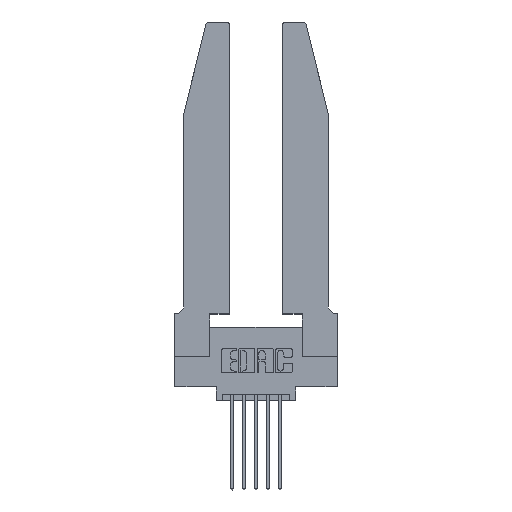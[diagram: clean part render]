
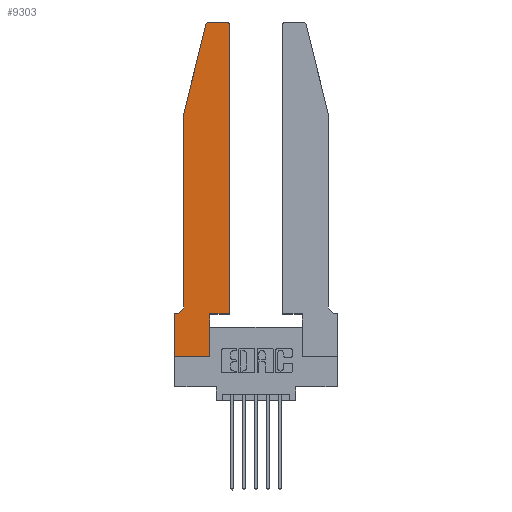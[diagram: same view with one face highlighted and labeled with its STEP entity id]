
A CAD part, top view. The second image highlights one B-rep face of the part: STEP entity #9303.
In plain terms, the highlighted planar face has unit normal (0, 0, 1).
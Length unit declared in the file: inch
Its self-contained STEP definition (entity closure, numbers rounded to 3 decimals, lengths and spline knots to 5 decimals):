
#86 = VECTOR ( 'NONE', #9740, 39.37008 ) ;
#114 = DIRECTION ( 'NONE',  ( 1., 0., 0. ) ) ;
#290 = AXIS2_PLACEMENT_3D ( 'NONE', #9185, #13426, #3967 ) ;
#351 = ORIENTED_EDGE ( 'NONE', *, *, #12800, .T. ) ;
#453 = DIRECTION ( 'NONE',  ( -0.239, -0.971, 0. ) ) ;
#692 = DIRECTION ( 'NONE',  ( -1., 0., 0. ) ) ;
#730 = DIRECTION ( 'NONE',  ( 0., 0., -1. ) ) ;
#731 = LINE ( 'NONE', #10114, #8862 ) ;
#1181 = EDGE_LOOP ( 'NONE', ( #2588, #9668, #1284, #3282, #1557, #1576, #5145, #13484, #11852, #12600, #351, #10222 ) ) ;
#1255 = VERTEX_POINT ( 'NONE', #8959 ) ;
#1274 = VECTOR ( 'NONE', #9961, 39.37008 ) ;
#1284 = ORIENTED_EDGE ( 'NONE', *, *, #6888, .T. ) ;
#1454 = VERTEX_POINT ( 'NONE', #12393 ) ;
#1557 = ORIENTED_EDGE ( 'NONE', *, *, #5245, .T. ) ;
#1576 = ORIENTED_EDGE ( 'NONE', *, *, #7895, .T. ) ;
#1739 = VERTEX_POINT ( 'NONE', #3591 ) ;
#1888 = CARTESIAN_POINT ( 'NONE',  ( 0.0755, 0.35, 0.37 ) ) ;
#1970 = EDGE_CURVE ( 'NONE', #13245, #1454, #8098, .T. ) ;
#2233 = DIRECTION ( 'NONE',  ( 0., 0., 1. ) ) ;
#2588 = ORIENTED_EDGE ( 'NONE', *, *, #2716, .T. ) ;
#2716 = EDGE_CURVE ( 'NONE', #13234, #9374, #2954, .T. ) ;
#2784 = LINE ( 'NONE', #7825, #5095 ) ;
#2932 = LINE ( 'NONE', #13042, #86 ) ;
#2954 = LINE ( 'NONE', #10415, #1274 ) ;
#3282 = ORIENTED_EDGE ( 'NONE', *, *, #12031, .T. ) ;
#3289 = EDGE_CURVE ( 'NONE', #9612, #13245, #2932, .T. ) ;
#3507 = AXIS2_PLACEMENT_3D ( 'NONE', #5927, #730, #692 ) ;
#3513 = CARTESIAN_POINT ( 'NONE',  ( 0.284, 2.75, 0.37 ) ) ;
#3564 = VECTOR ( 'NONE', #13738, 39.37008 ) ;
#3591 = CARTESIAN_POINT ( 'NONE',  ( 0.4505, 2.72, 0.37 ) ) ;
#3671 = CARTESIAN_POINT ( 'NONE',  ( 0.0755, 2., 0.37 ) ) ;
#3807 = VECTOR ( 'NONE', #8045, 39.37008 ) ;
#3967 = DIRECTION ( 'NONE',  ( 1., 0., 0. ) ) ;
#4222 = DIRECTION ( 'NONE',  ( -1., 0., 0. ) ) ;
#4382 = EDGE_CURVE ( 'NONE', #9374, #4747, #5225, .T. ) ;
#4434 = LINE ( 'NONE', #7613, #11574 ) ;
#4711 = VECTOR ( 'NONE', #4222, 39.37008 ) ;
#4747 = VERTEX_POINT ( 'NONE', #6871 ) ;
#4800 = CARTESIAN_POINT ( 'NONE',  ( 0.0055, 0.35, 0.37 ) ) ;
#4883 = CIRCLE ( 'NONE', #12357, 0.03 ) ;
#4954 = CARTESIAN_POINT ( 'NONE',  ( 0.4505, 0.35, 0.37 ) ) ;
#5095 = VECTOR ( 'NONE', #7964, 39.37008 ) ;
#5145 = ORIENTED_EDGE ( 'NONE', *, *, #7272, .T. ) ;
#5225 = CIRCLE ( 'NONE', #290, 0.03 ) ;
#5245 = EDGE_CURVE ( 'NONE', #10984, #12895, #6086, .T. ) ;
#5383 = LINE ( 'NONE', #3671, #7863 ) ;
#5430 = DIRECTION ( 'NONE',  ( 0., -1., 0. ) ) ;
#5453 = CARTESIAN_POINT ( 'NONE',  ( 0.0755, 0.42, 0.37 ) ) ;
#5628 = EDGE_CURVE ( 'NONE', #9813, #9612, #2784, .T. ) ;
#5927 = CARTESIAN_POINT ( 'NONE',  ( 0.0055, 0.42, 0.37 ) ) ;
#6086 = CIRCLE ( 'NONE', #3507, 0.07 ) ;
#6871 = CARTESIAN_POINT ( 'NONE',  ( 0.25487, 2.72718, 0.37 ) ) ;
#6888 = EDGE_CURVE ( 'NONE', #4747, #1255, #5383, .T. ) ;
#6935 = CARTESIAN_POINT ( 'NONE',  ( 0.4205, 2.75, 0.37 ) ) ;
#7025 = DIRECTION ( 'NONE',  ( 1., 0., 0. ) ) ;
#7216 = CARTESIAN_POINT ( 'NONE',  ( 0.2865, 0., 0.37 ) ) ;
#7272 = EDGE_CURVE ( 'NONE', #12664, #9813, #13235, .T. ) ;
#7532 = LINE ( 'NONE', #1888, #4711 ) ;
#7613 = CARTESIAN_POINT ( 'NONE',  ( 0.0755, 2., 0.37 ) ) ;
#7825 = CARTESIAN_POINT ( 'NONE',  ( 0., 0., 0.37 ) ) ;
#7863 = VECTOR ( 'NONE', #453, 39.37008 ) ;
#7895 = EDGE_CURVE ( 'NONE', #12895, #12664, #7532, .T. ) ;
#7964 = DIRECTION ( 'NONE',  ( 1., 0., 0. ) ) ;
#8045 = DIRECTION ( 'NONE',  ( 1., 0., 0. ) ) ;
#8098 = LINE ( 'NONE', #4954, #3807 ) ;
#8421 = CARTESIAN_POINT ( 'NONE',  ( 0., 0., 0.37 ) ) ;
#8565 = CARTESIAN_POINT ( 'NONE',  ( 0., 0.35, 0.37 ) ) ;
#8602 = CARTESIAN_POINT ( 'NONE',  ( 0., 0.35, 0.37 ) ) ;
#8862 = VECTOR ( 'NONE', #12236, 39.37008 ) ;
#8959 = CARTESIAN_POINT ( 'NONE',  ( 0.0755, 2., 0.37 ) ) ;
#9185 = CARTESIAN_POINT ( 'NONE',  ( 0.284, 2.72, 0.37 ) ) ;
#9290 = CARTESIAN_POINT ( 'NONE',  ( 0.4205, 2.72, 0.37 ) ) ;
#9303 = ADVANCED_FACE ( 'NONE', ( #13374 ), #12839, .T. ) ;
#9374 = VERTEX_POINT ( 'NONE', #3513 ) ;
#9436 = CARTESIAN_POINT ( 'NONE',  ( 0., 0., 0.37 ) ) ;
#9612 = VERTEX_POINT ( 'NONE', #7216 ) ;
#9668 = ORIENTED_EDGE ( 'NONE', *, *, #4382, .T. ) ;
#9740 = DIRECTION ( 'NONE',  ( 0., 1., 0. ) ) ;
#9813 = VERTEX_POINT ( 'NONE', #9436 ) ;
#9961 = DIRECTION ( 'NONE',  ( -1., 0., 0. ) ) ;
#10114 = CARTESIAN_POINT ( 'NONE',  ( 0.4505, 0.35, 0.37 ) ) ;
#10222 = ORIENTED_EDGE ( 'NONE', *, *, #13287, .T. ) ;
#10415 = CARTESIAN_POINT ( 'NONE',  ( 0.2605, 2.75, 0.37 ) ) ;
#10984 = VERTEX_POINT ( 'NONE', #5453 ) ;
#11127 = CARTESIAN_POINT ( 'NONE',  ( 0.2865, 0.35, 0.37 ) ) ;
#11268 = DIRECTION ( 'NONE',  ( 0., 0., 1. ) ) ;
#11574 = VECTOR ( 'NONE', #5430, 39.37008 ) ;
#11852 = ORIENTED_EDGE ( 'NONE', *, *, #3289, .T. ) ;
#12031 = EDGE_CURVE ( 'NONE', #1255, #10984, #4434, .T. ) ;
#12236 = DIRECTION ( 'NONE',  ( 0., 1., 0. ) ) ;
#12357 = AXIS2_PLACEMENT_3D ( 'NONE', #9290, #11268, #7025 ) ;
#12393 = CARTESIAN_POINT ( 'NONE',  ( 0.4505, 0.35, 0.37 ) ) ;
#12600 = ORIENTED_EDGE ( 'NONE', *, *, #1970, .T. ) ;
#12664 = VERTEX_POINT ( 'NONE', #8602 ) ;
#12800 = EDGE_CURVE ( 'NONE', #1454, #1739, #731, .T. ) ;
#12839 = PLANE ( 'NONE',  #13420 ) ;
#12895 = VERTEX_POINT ( 'NONE', #4800 ) ;
#13042 = CARTESIAN_POINT ( 'NONE',  ( 0.2865, 0.35, 0.37 ) ) ;
#13234 = VERTEX_POINT ( 'NONE', #6935 ) ;
#13235 = LINE ( 'NONE', #8421, #3564 ) ;
#13245 = VERTEX_POINT ( 'NONE', #11127 ) ;
#13287 = EDGE_CURVE ( 'NONE', #1739, #13234, #4883, .T. ) ;
#13374 = FACE_OUTER_BOUND ( 'NONE', #1181, .T. ) ;
#13420 = AXIS2_PLACEMENT_3D ( 'NONE', #8565, #2233, #114 ) ;
#13426 = DIRECTION ( 'NONE',  ( 0., 0., 1. ) ) ;
#13484 = ORIENTED_EDGE ( 'NONE', *, *, #5628, .T. ) ;
#13738 = DIRECTION ( 'NONE',  ( 0., -1., 0. ) ) ;
